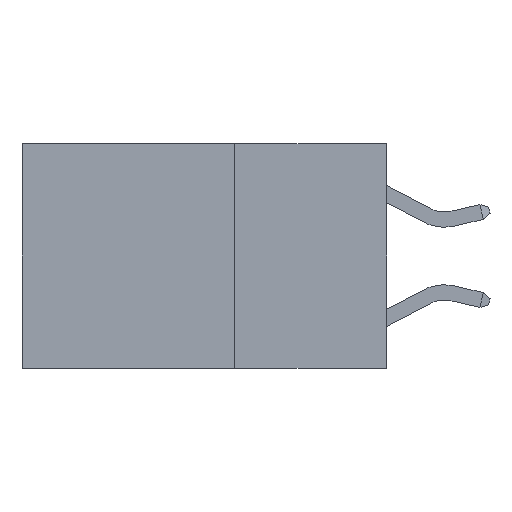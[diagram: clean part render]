
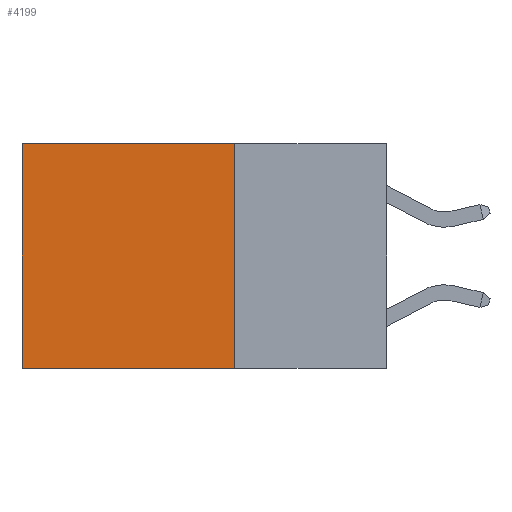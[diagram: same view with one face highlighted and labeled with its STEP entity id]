
A CAD part, left-side view. The second image highlights one B-rep face of the part: STEP entity #4199.
In plain terms, the highlighted planar face has unit normal (-1, 0, 0).
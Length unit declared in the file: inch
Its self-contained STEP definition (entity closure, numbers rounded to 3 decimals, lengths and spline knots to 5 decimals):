
#68 = DIRECTION ( 'NONE',  ( 1., 0., 0. ) ) ;
#183 = LINE ( 'NONE', #4502, #2345 ) ;
#350 = EDGE_CURVE ( 'NONE', #714, #3399, #3899, .T. ) ;
#714 = VERTEX_POINT ( 'NONE', #3814 ) ;
#888 = EDGE_LOOP ( 'NONE', ( #3833, #2643, #7295, #1549 ) ) ;
#1549 = ORIENTED_EDGE ( 'NONE', *, *, #5303, .T. ) ;
#1747 = DIRECTION ( 'NONE',  ( 0., 1., 0. ) ) ;
#2345 = VECTOR ( 'NONE', #2877, 39.37008 ) ;
#2643 = ORIENTED_EDGE ( 'NONE', *, *, #350, .F. ) ;
#2824 = DIRECTION ( 'NONE',  ( 0., 0., -1. ) ) ;
#2877 = DIRECTION ( 'NONE',  ( 0., 0., -1. ) ) ;
#3154 = CARTESIAN_POINT ( 'NONE',  ( 0.2625, 0.6, -0.37 ) ) ;
#3180 = DIRECTION ( 'NONE',  ( 0., 1., 0. ) ) ;
#3399 = VERTEX_POINT ( 'NONE', #3154 ) ;
#3814 = CARTESIAN_POINT ( 'NONE',  ( 0.2625, 0.25, -0.37 ) ) ;
#3833 = ORIENTED_EDGE ( 'NONE', *, *, #10221, .T. ) ;
#3899 = LINE ( 'NONE', #5896, #8953 ) ;
#4199 = ADVANCED_FACE ( 'NONE', ( #7250 ), #4608, .F. ) ;
#4502 = CARTESIAN_POINT ( 'NONE',  ( 0.2625, 0.6, 0. ) ) ;
#4608 = PLANE ( 'NONE',  #10490 ) ;
#4612 = VERTEX_POINT ( 'NONE', #9027 ) ;
#5047 = VECTOR ( 'NONE', #10656, 39.37008 ) ;
#5232 = VERTEX_POINT ( 'NONE', #8157 ) ;
#5248 = LINE ( 'NONE', #7720, #5047 ) ;
#5303 = EDGE_CURVE ( 'NONE', #4612, #5232, #5622, .T. ) ;
#5622 = LINE ( 'NONE', #6268, #7829 ) ;
#5896 = CARTESIAN_POINT ( 'NONE',  ( 0.2625, 0.25, -0.37 ) ) ;
#6268 = CARTESIAN_POINT ( 'NONE',  ( 0.2625, 0.25, 0. ) ) ;
#7250 = FACE_OUTER_BOUND ( 'NONE', #888, .T. ) ;
#7295 = ORIENTED_EDGE ( 'NONE', *, *, #7576, .F. ) ;
#7576 = EDGE_CURVE ( 'NONE', #4612, #714, #5248, .T. ) ;
#7720 = CARTESIAN_POINT ( 'NONE',  ( 0.2625, 0.25, 0. ) ) ;
#7829 = VECTOR ( 'NONE', #1747, 39.37008 ) ;
#8157 = CARTESIAN_POINT ( 'NONE',  ( 0.2625, 0.6, 0. ) ) ;
#8953 = VECTOR ( 'NONE', #3180, 39.37008 ) ;
#9027 = CARTESIAN_POINT ( 'NONE',  ( 0.2625, 0.25, 0. ) ) ;
#10221 = EDGE_CURVE ( 'NONE', #5232, #3399, #183, .T. ) ;
#10490 = AXIS2_PLACEMENT_3D ( 'NONE', #10901, #68, #2824 ) ;
#10656 = DIRECTION ( 'NONE',  ( 0., 0., -1. ) ) ;
#10901 = CARTESIAN_POINT ( 'NONE',  ( 0.2625, 0.25, 0. ) ) ;
